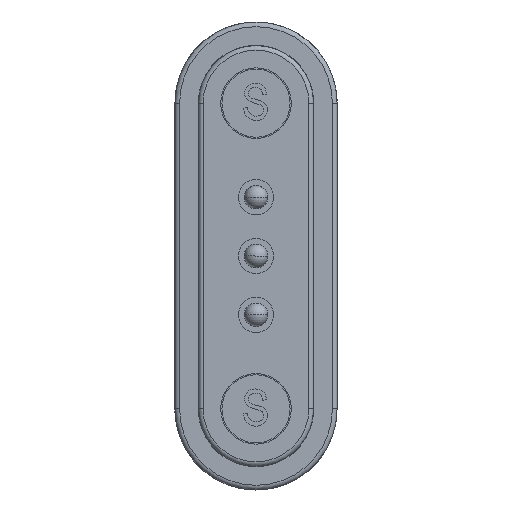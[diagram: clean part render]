
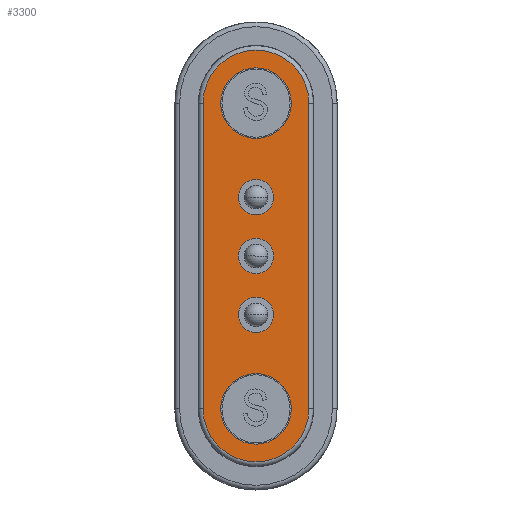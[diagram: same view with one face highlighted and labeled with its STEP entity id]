
A CAD part, front view. The second image highlights one B-rep face of the part: STEP entity #3300.
In plain terms, the highlighted planar face has unit normal (0, -1, 0).
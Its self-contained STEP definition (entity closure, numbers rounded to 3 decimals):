
#8 = LINE ( 'NONE', #2588, #1916 ) ;
#62 = EDGE_CURVE ( 'NONE', #3745, #6182, #6319, .T. ) ;
#101 = EDGE_LOOP ( 'NONE', ( #7148, #1294 ) ) ;
#120 = VERTEX_POINT ( 'NONE', #2516 ) ;
#199 = FACE_OUTER_BOUND ( 'NONE', #4232, .T. ) ;
#258 = CIRCLE ( 'NONE', #515, 1.5 ) ;
#263 = EDGE_CURVE ( 'NONE', #7706, #1913, #7685, .T. ) ;
#268 = CARTESIAN_POINT ( 'NONE',  ( 2.5, 22.74, 0.75 ) ) ;
#462 = AXIS2_PLACEMENT_3D ( 'NONE', #5025, #7647, #1785 ) ;
#493 = DIRECTION ( 'NONE',  ( 0., -1., 0. ) ) ;
#515 = AXIS2_PLACEMENT_3D ( 'NONE', #4958, #7582, #1721 ) ;
#719 = AXIS2_PLACEMENT_3D ( 'NONE', #6326, #493, #3065 ) ;
#856 = VECTOR ( 'NONE', #3703, 1000. ) ;
#874 = AXIS2_PLACEMENT_3D ( 'NONE', #4738, #7358, #1501 ) ;
#919 = VERTEX_POINT ( 'NONE', #7186 ) ;
#1029 = ORIENTED_EDGE ( 'NONE', *, *, #7828, .F. ) ;
#1120 = CARTESIAN_POINT ( 'NONE',  ( 4.748, 22.74, -6.5 ) ) ;
#1185 = CARTESIAN_POINT ( 'NONE',  ( 2.5, 22.74, 8. ) ) ;
#1208 = DIRECTION ( 'NONE',  ( 1., 0., -0.018 ) ) ;
#1256 = CARTESIAN_POINT ( 'NONE',  ( 2.5, 22.74, 0. ) ) ;
#1294 = ORIENTED_EDGE ( 'NONE', *, *, #263, .F. ) ;
#1349 = CIRCLE ( 'NONE', #5984, 1.5 ) ;
#1374 = CARTESIAN_POINT ( 'NONE',  ( 2.5, 22.74, 2.5 ) ) ;
#1424 = EDGE_LOOP ( 'NONE', ( #1029, #8083 ) ) ;
#1465 = DIRECTION ( 'NONE',  ( 1., 0., 0. ) ) ;
#1501 = DIRECTION ( 'NONE',  ( 1., 0., 0. ) ) ;
#1512 = DIRECTION ( 'NONE',  ( -1., 0., 0.018 ) ) ;
#1633 = EDGE_CURVE ( 'NONE', #2898, #6223, #8, .T. ) ;
#1721 = DIRECTION ( 'NONE',  ( 0., 0., -1. ) ) ;
#1744 = VERTEX_POINT ( 'NONE', #4804 ) ;
#1785 = DIRECTION ( 'NONE',  ( 0., 0., -1. ) ) ;
#1892 = CIRCLE ( 'NONE', #2978, 0.75 ) ;
#1913 = VERTEX_POINT ( 'NONE', #2537 ) ;
#1916 = VECTOR ( 'NONE', #5181, 1000. ) ;
#1980 = EDGE_CURVE ( 'NONE', #6551, #120, #5029, .T. ) ;
#2021 = DIRECTION ( 'NONE',  ( 0., -1., 0. ) ) ;
#2055 = DIRECTION ( 'NONE',  ( 0., 0., -1. ) ) ;
#2072 = CIRCLE ( 'NONE', #719, 0.75 ) ;
#2146 = PLANE ( 'NONE',  #874 ) ;
#2245 = CARTESIAN_POINT ( 'NONE',  ( 2.5, 22.74, -2.5 ) ) ;
#2278 = CARTESIAN_POINT ( 'NONE',  ( 0.252, 22.74, 6.5 ) ) ;
#2516 = CARTESIAN_POINT ( 'NONE',  ( 2.5, 22.74, -0.75 ) ) ;
#2537 = CARTESIAN_POINT ( 'NONE',  ( 1.75, 22.74, -2.5 ) ) ;
#2539 = VERTEX_POINT ( 'NONE', #4466 ) ;
#2582 = CARTESIAN_POINT ( 'NONE',  ( 2.5, 22.74, 6.5 ) ) ;
#2588 = CARTESIAN_POINT ( 'NONE',  ( 0.252, 22.74, 6.5 ) ) ;
#2777 = FACE_BOUND ( 'NONE', #8408, .T. ) ;
#2827 = EDGE_CURVE ( 'NONE', #919, #2898, #5215, .T. ) ;
#2873 = AXIS2_PLACEMENT_3D ( 'NONE', #4440, #7067, #1208 ) ;
#2898 = VERTEX_POINT ( 'NONE', #2278 ) ;
#2978 = AXIS2_PLACEMENT_3D ( 'NONE', #1256, #3848, #6469 ) ;
#3001 = CIRCLE ( 'NONE', #7407, 0.75 ) ;
#3012 = AXIS2_PLACEMENT_3D ( 'NONE', #2582, #5176, #7804 ) ;
#3065 = DIRECTION ( 'NONE',  ( -1., 0., 0. ) ) ;
#3126 = ORIENTED_EDGE ( 'NONE', *, *, #1980, .F. ) ;
#3274 = CIRCLE ( 'NONE', #3012, 1.5 ) ;
#3300 = ADVANCED_FACE ( 'NONE', ( #3398, #6023, #199, #2777, #5371, #8001 ), #2146, .F. ) ;
#3398 = FACE_BOUND ( 'NONE', #7069, .T. ) ;
#3497 = EDGE_CURVE ( 'NONE', #6223, #3940, #8215, .T. ) ;
#3703 = DIRECTION ( 'NONE',  ( 0., 0., 1. ) ) ;
#3745 = VERTEX_POINT ( 'NONE', #1185 ) ;
#3848 = DIRECTION ( 'NONE',  ( 0., -1., 0. ) ) ;
#3860 = ORIENTED_EDGE ( 'NONE', *, *, #6931, .F. ) ;
#3940 = VERTEX_POINT ( 'NONE', #6563 ) ;
#3968 = DIRECTION ( 'NONE',  ( 0., -1., 0. ) ) ;
#4043 = ORIENTED_EDGE ( 'NONE', *, *, #7522, .F. ) ;
#4084 = CIRCLE ( 'NONE', #4613, 0.75 ) ;
#4232 = EDGE_LOOP ( 'NONE', ( #6167, #6815, #5424, #5144 ) ) ;
#4440 = CARTESIAN_POINT ( 'NONE',  ( 2.5, 22.74, -6.5 ) ) ;
#4466 = CARTESIAN_POINT ( 'NONE',  ( 1.75, 22.74, 2.5 ) ) ;
#4613 = AXIS2_PLACEMENT_3D ( 'NONE', #4700, #7326, #1465 ) ;
#4617 = DIRECTION ( 'NONE',  ( 0., 0., 1. ) ) ;
#4629 = ORIENTED_EDGE ( 'NONE', *, *, #5095, .F. ) ;
#4637 = VERTEX_POINT ( 'NONE', #8096 ) ;
#4700 = CARTESIAN_POINT ( 'NONE',  ( 2.5, 22.74, 2.5 ) ) ;
#4738 = CARTESIAN_POINT ( 'NONE',  ( 2.5, 22.74, 0. ) ) ;
#4748 = CARTESIAN_POINT ( 'NONE',  ( 2.5, 22.74, 6.5 ) ) ;
#4804 = CARTESIAN_POINT ( 'NONE',  ( 2.5, 22.74, -8. ) ) ;
#4842 = DIRECTION ( 'NONE',  ( 0., -1., 0. ) ) ;
#4932 = EDGE_CURVE ( 'NONE', #6269, #2539, #4084, .T. ) ;
#4958 = CARTESIAN_POINT ( 'NONE',  ( 2.5, 22.74, -6.5 ) ) ;
#4993 = CARTESIAN_POINT ( 'NONE',  ( 2.5, 22.74, 5. ) ) ;
#5025 = CARTESIAN_POINT ( 'NONE',  ( 2.5, 22.74, 6.5 ) ) ;
#5029 = CIRCLE ( 'NONE', #7500, 0.75 ) ;
#5095 = EDGE_CURVE ( 'NONE', #120, #6551, #1892, .T. ) ;
#5144 = ORIENTED_EDGE ( 'NONE', *, *, #3497, .T. ) ;
#5176 = DIRECTION ( 'NONE',  ( 0., -1., 0. ) ) ;
#5181 = DIRECTION ( 'NONE',  ( 0., 0., -1. ) ) ;
#5215 = CIRCLE ( 'NONE', #5464, 2.248 ) ;
#5236 = EDGE_CURVE ( 'NONE', #4637, #1744, #1349, .T. ) ;
#5285 = CARTESIAN_POINT ( 'NONE',  ( 2.5, 22.74, -6.5 ) ) ;
#5371 = FACE_BOUND ( 'NONE', #5722, .T. ) ;
#5424 = ORIENTED_EDGE ( 'NONE', *, *, #1633, .T. ) ;
#5464 = AXIS2_PLACEMENT_3D ( 'NONE', #4748, #7371, #1512 ) ;
#5722 = EDGE_LOOP ( 'NONE', ( #3126, #4629 ) ) ;
#5741 = ORIENTED_EDGE ( 'NONE', *, *, #62, .F. ) ;
#5984 = AXIS2_PLACEMENT_3D ( 'NONE', #5285, #7910, #2055 ) ;
#6023 = FACE_BOUND ( 'NONE', #1424, .T. ) ;
#6066 = ORIENTED_EDGE ( 'NONE', *, *, #4932, .F. ) ;
#6113 = CARTESIAN_POINT ( 'NONE',  ( 3.25, 22.74, -2.5 ) ) ;
#6167 = ORIENTED_EDGE ( 'NONE', *, *, #6191, .T. ) ;
#6182 = VERTEX_POINT ( 'NONE', #4993 ) ;
#6191 = EDGE_CURVE ( 'NONE', #3940, #919, #6971, .T. ) ;
#6199 = EDGE_CURVE ( 'NONE', #1913, #7706, #2072, .T. ) ;
#6223 = VERTEX_POINT ( 'NONE', #7021 ) ;
#6269 = VERTEX_POINT ( 'NONE', #7741 ) ;
#6319 = CIRCLE ( 'NONE', #462, 1.5 ) ;
#6326 = CARTESIAN_POINT ( 'NONE',  ( 2.5, 22.74, -2.5 ) ) ;
#6469 = DIRECTION ( 'NONE',  ( 0., 0., -1. ) ) ;
#6551 = VERTEX_POINT ( 'NONE', #268 ) ;
#6563 = CARTESIAN_POINT ( 'NONE',  ( 4.748, 22.74, -6.5 ) ) ;
#6598 = DIRECTION ( 'NONE',  ( -1., 0., 0. ) ) ;
#6815 = ORIENTED_EDGE ( 'NONE', *, *, #2827, .T. ) ;
#6931 = EDGE_CURVE ( 'NONE', #2539, #6269, #3001, .T. ) ;
#6971 = LINE ( 'NONE', #1120, #856 ) ;
#7021 = CARTESIAN_POINT ( 'NONE',  ( 0.252, 22.74, -6.5 ) ) ;
#7067 = DIRECTION ( 'NONE',  ( 0., -1., 0. ) ) ;
#7069 = EDGE_LOOP ( 'NONE', ( #4043, #5741 ) ) ;
#7148 = ORIENTED_EDGE ( 'NONE', *, *, #6199, .F. ) ;
#7186 = CARTESIAN_POINT ( 'NONE',  ( 4.748, 22.74, 6.5 ) ) ;
#7326 = DIRECTION ( 'NONE',  ( 0., -1., 0. ) ) ;
#7358 = DIRECTION ( 'NONE',  ( 0., 1., 0. ) ) ;
#7371 = DIRECTION ( 'NONE',  ( 0., -1., 0. ) ) ;
#7404 = AXIS2_PLACEMENT_3D ( 'NONE', #2245, #4842, #7461 ) ;
#7407 = AXIS2_PLACEMENT_3D ( 'NONE', #1374, #3968, #6598 ) ;
#7461 = DIRECTION ( 'NONE',  ( 1., 0., 0. ) ) ;
#7500 = AXIS2_PLACEMENT_3D ( 'NONE', #7879, #2021, #4617 ) ;
#7522 = EDGE_CURVE ( 'NONE', #6182, #3745, #3274, .T. ) ;
#7582 = DIRECTION ( 'NONE',  ( 0., -1., 0. ) ) ;
#7647 = DIRECTION ( 'NONE',  ( 0., -1., 0. ) ) ;
#7685 = CIRCLE ( 'NONE', #7404, 0.75 ) ;
#7706 = VERTEX_POINT ( 'NONE', #6113 ) ;
#7741 = CARTESIAN_POINT ( 'NONE',  ( 3.25, 22.74, 2.5 ) ) ;
#7804 = DIRECTION ( 'NONE',  ( 0., 0., -1. ) ) ;
#7828 = EDGE_CURVE ( 'NONE', #1744, #4637, #258, .T. ) ;
#7879 = CARTESIAN_POINT ( 'NONE',  ( 2.5, 22.74, 0. ) ) ;
#7910 = DIRECTION ( 'NONE',  ( 0., -1., 0. ) ) ;
#8001 = FACE_BOUND ( 'NONE', #101, .T. ) ;
#8083 = ORIENTED_EDGE ( 'NONE', *, *, #5236, .F. ) ;
#8096 = CARTESIAN_POINT ( 'NONE',  ( 2.5, 22.74, -5. ) ) ;
#8215 = CIRCLE ( 'NONE', #2873, 2.248 ) ;
#8408 = EDGE_LOOP ( 'NONE', ( #3860, #6066 ) ) ;
